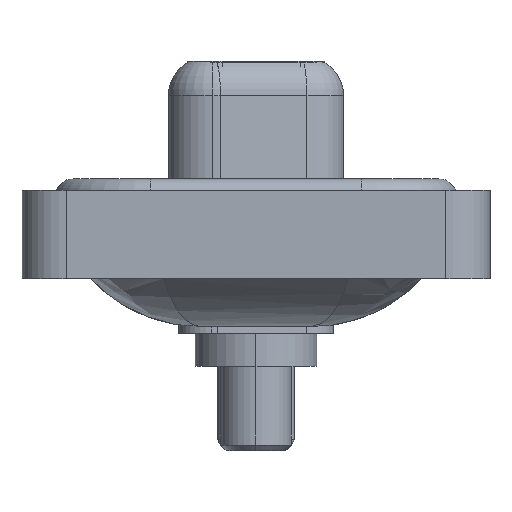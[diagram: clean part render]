
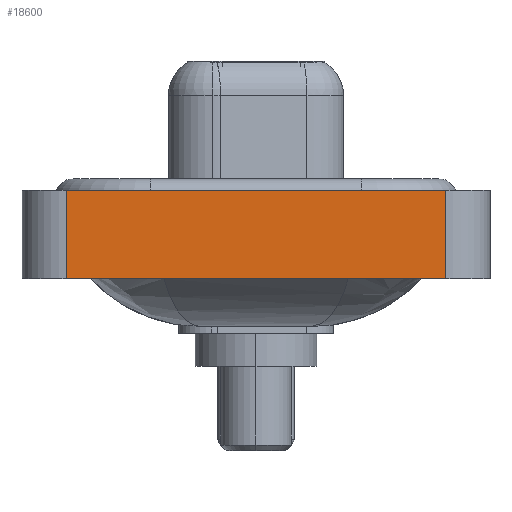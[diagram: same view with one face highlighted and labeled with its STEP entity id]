
A CAD part, left-side view. The second image highlights one B-rep face of the part: STEP entity #18600.
In plain terms, the highlighted planar face has unit normal (-1, 0, 0).
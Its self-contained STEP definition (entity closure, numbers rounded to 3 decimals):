
#1557 = CARTESIAN_POINT ( 'NONE',  ( -7.35, -8.55, 0.4 ) ) ;
#1844 = LINE ( 'NONE', #10872, #9812 ) ;
#2229 = CARTESIAN_POINT ( 'NONE',  ( -7.35, 8.55, -3.6 ) ) ;
#3140 = DIRECTION ( 'NONE',  ( 0., 0., 1. ) ) ;
#3245 = DIRECTION ( 'NONE',  ( 0., 0., 1. ) ) ;
#3416 = LINE ( 'NONE', #10342, #9898 ) ;
#3427 = EDGE_CURVE ( 'NONE', #4490, #5867, #10066, .T. ) ;
#4163 = EDGE_CURVE ( 'NONE', #12945, #4490, #5395, .T. ) ;
#4490 = VERTEX_POINT ( 'NONE', #22544 ) ;
#4609 = ORIENTED_EDGE ( 'NONE', *, *, #3427, .T. ) ;
#4852 = VERTEX_POINT ( 'NONE', #20748 ) ;
#5194 = CARTESIAN_POINT ( 'NONE',  ( -7.35, -8.55, -3.6 ) ) ;
#5395 = LINE ( 'NONE', #19560, #11354 ) ;
#5867 = VERTEX_POINT ( 'NONE', #1557 ) ;
#7407 = EDGE_CURVE ( 'NONE', #12945, #4852, #1844, .T. ) ;
#7513 = ORIENTED_EDGE ( 'NONE', *, *, #7407, .F. ) ;
#9812 = VECTOR ( 'NONE', #10519, 1000. ) ;
#9898 = VECTOR ( 'NONE', #12296, 1000. ) ;
#10066 = LINE ( 'NONE', #17437, #20502 ) ;
#10172 = DIRECTION ( 'NONE',  ( -1., 0., 0. ) ) ;
#10342 = CARTESIAN_POINT ( 'NONE',  ( -7.35, -8.55, 0.4 ) ) ;
#10519 = DIRECTION ( 'NONE',  ( 0., 0., 1. ) ) ;
#10872 = CARTESIAN_POINT ( 'NONE',  ( -7.35, 8.55, -3.6 ) ) ;
#11354 = VECTOR ( 'NONE', #12315, 1000. ) ;
#12296 = DIRECTION ( 'NONE',  ( 0., -1., 0. ) ) ;
#12315 = DIRECTION ( 'NONE',  ( 0., -1., 0. ) ) ;
#12945 = VERTEX_POINT ( 'NONE', #2229 ) ;
#14935 = ORIENTED_EDGE ( 'NONE', *, *, #4163, .T. ) ;
#15688 = PLANE ( 'NONE',  #15904 ) ;
#15904 = AXIS2_PLACEMENT_3D ( 'NONE', #5194, #10172, #3245 ) ;
#16340 = ORIENTED_EDGE ( 'NONE', *, *, #19502, .F. ) ;
#17437 = CARTESIAN_POINT ( 'NONE',  ( -7.35, -8.55, -3.6 ) ) ;
#18600 = ADVANCED_FACE ( 'NONE', ( #20755 ), #15688, .T. ) ;
#18652 = EDGE_LOOP ( 'NONE', ( #4609, #16340, #7513, #14935 ) ) ;
#19502 = EDGE_CURVE ( 'NONE', #4852, #5867, #3416, .T. ) ;
#19560 = CARTESIAN_POINT ( 'NONE',  ( -7.35, -8.55, -3.6 ) ) ;
#20502 = VECTOR ( 'NONE', #3140, 1000. ) ;
#20748 = CARTESIAN_POINT ( 'NONE',  ( -7.35, 8.55, 0.4 ) ) ;
#20755 = FACE_OUTER_BOUND ( 'NONE', #18652, .T. ) ;
#22544 = CARTESIAN_POINT ( 'NONE',  ( -7.35, -8.55, -3.6 ) ) ;
